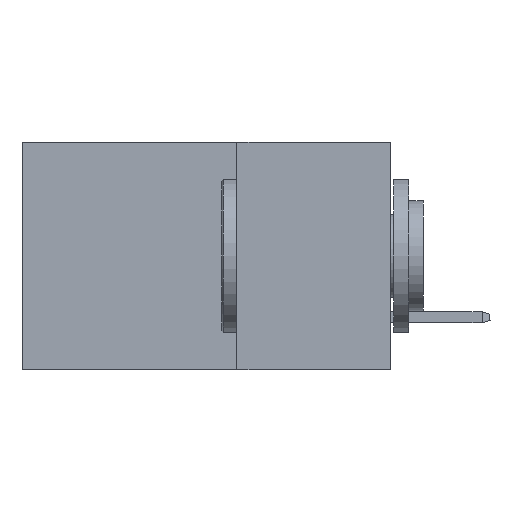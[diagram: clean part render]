
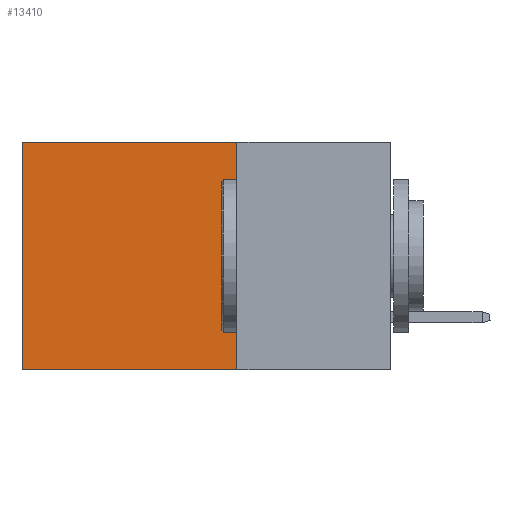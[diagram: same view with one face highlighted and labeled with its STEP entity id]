
A CAD part, left-side view. The second image highlights one B-rep face of the part: STEP entity #13410.
In plain terms, the highlighted planar face has unit normal (-1, 0, 0).
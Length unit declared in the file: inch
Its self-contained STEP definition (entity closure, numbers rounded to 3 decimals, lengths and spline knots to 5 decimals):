
#615 = CARTESIAN_POINT ( 'NONE',  ( 0.2875, 0.25, -0.37 ) ) ;
#676 = EDGE_CURVE ( 'NONE', #1327, #6812, #2978, .T. ) ;
#740 = LINE ( 'NONE', #7591, #16373 ) ;
#1327 = VERTEX_POINT ( 'NONE', #14099 ) ;
#1645 = ORIENTED_EDGE ( 'NONE', *, *, #676, .F. ) ;
#2978 = LINE ( 'NONE', #9778, #5283 ) ;
#3484 = DIRECTION ( 'NONE',  ( 0., 0., -1. ) ) ;
#3780 = VECTOR ( 'NONE', #16757, 39.37008 ) ;
#3802 = EDGE_CURVE ( 'NONE', #6812, #9607, #4715, .T. ) ;
#3817 = AXIS2_PLACEMENT_3D ( 'NONE', #9267, #12204, #3484 ) ;
#4134 = DIRECTION ( 'NONE',  ( 0., 0., -1. ) ) ;
#4715 = LINE ( 'NONE', #8429, #3780 ) ;
#5283 = VECTOR ( 'NONE', #4134, 39.37008 ) ;
#6812 = VERTEX_POINT ( 'NONE', #615 ) ;
#7133 = VECTOR ( 'NONE', #17987, 39.37008 ) ;
#7591 = CARTESIAN_POINT ( 'NONE',  ( 0.2875, 0.25, 0. ) ) ;
#7670 = VERTEX_POINT ( 'NONE', #12660 ) ;
#8429 = CARTESIAN_POINT ( 'NONE',  ( 0.2875, 0.25, -0.37 ) ) ;
#8759 = EDGE_CURVE ( 'NONE', #7670, #9607, #11219, .T. ) ;
#9267 = CARTESIAN_POINT ( 'NONE',  ( 0.2875, 0.25, 0. ) ) ;
#9607 = VERTEX_POINT ( 'NONE', #10886 ) ;
#9778 = CARTESIAN_POINT ( 'NONE',  ( 0.2875, 0.25, 0. ) ) ;
#10886 = CARTESIAN_POINT ( 'NONE',  ( 0.2875, 0.6, -0.37 ) ) ;
#11219 = LINE ( 'NONE', #15166, #7133 ) ;
#11643 = ORIENTED_EDGE ( 'NONE', *, *, #3802, .F. ) ;
#12084 = PLANE ( 'NONE',  #3817 ) ;
#12204 = DIRECTION ( 'NONE',  ( 1., 0., 0. ) ) ;
#12660 = CARTESIAN_POINT ( 'NONE',  ( 0.2875, 0.6, 0. ) ) ;
#13049 = EDGE_LOOP ( 'NONE', ( #16334, #11643, #1645, #16471 ) ) ;
#13410 = ADVANCED_FACE ( 'NONE', ( #15318 ), #12084, .F. ) ;
#13749 = DIRECTION ( 'NONE',  ( 0., 1., 0. ) ) ;
#14099 = CARTESIAN_POINT ( 'NONE',  ( 0.2875, 0.25, 0. ) ) ;
#15166 = CARTESIAN_POINT ( 'NONE',  ( 0.2875, 0.6, 0. ) ) ;
#15318 = FACE_OUTER_BOUND ( 'NONE', #13049, .T. ) ;
#16334 = ORIENTED_EDGE ( 'NONE', *, *, #8759, .T. ) ;
#16373 = VECTOR ( 'NONE', #13749, 39.37008 ) ;
#16471 = ORIENTED_EDGE ( 'NONE', *, *, #18080, .T. ) ;
#16757 = DIRECTION ( 'NONE',  ( 0., 1., 0. ) ) ;
#17987 = DIRECTION ( 'NONE',  ( 0., 0., -1. ) ) ;
#18080 = EDGE_CURVE ( 'NONE', #1327, #7670, #740, .T. ) ;
